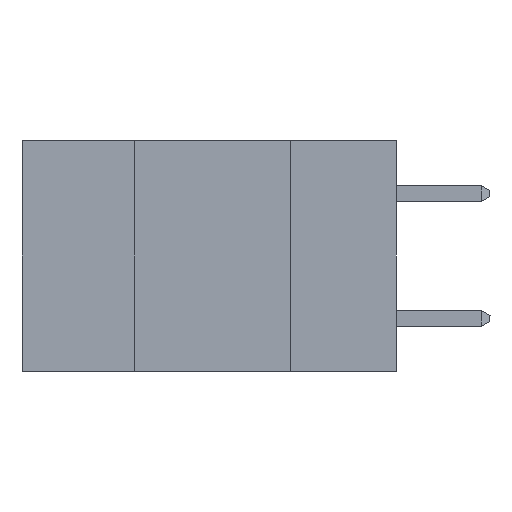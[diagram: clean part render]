
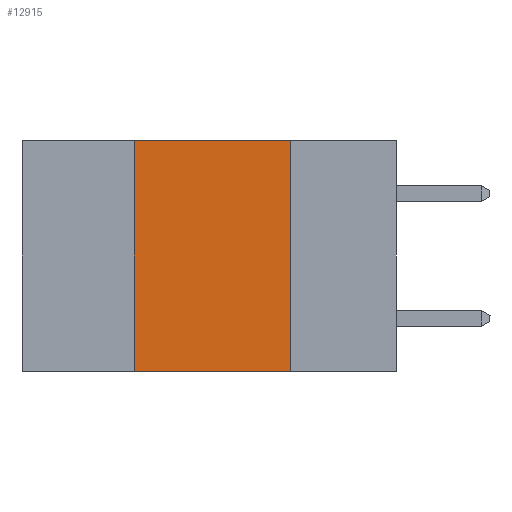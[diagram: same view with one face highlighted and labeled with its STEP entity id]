
A CAD part, left-side view. The second image highlights one B-rep face of the part: STEP entity #12915.
In plain terms, the highlighted planar face has unit normal (-1, 0, 0).
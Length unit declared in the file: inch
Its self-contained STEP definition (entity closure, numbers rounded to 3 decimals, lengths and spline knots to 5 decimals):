
#560 = LINE ( 'NONE', #1571, #10135 ) ;
#811 = LINE ( 'NONE', #8691, #4761 ) ;
#1571 = CARTESIAN_POINT ( 'NONE',  ( 0., 0.17, -0.37 ) ) ;
#2746 = CARTESIAN_POINT ( 'NONE',  ( 0., 0.42, -0.37 ) ) ;
#2854 = CARTESIAN_POINT ( 'NONE',  ( 0., 0.6, 0. ) ) ;
#3634 = CARTESIAN_POINT ( 'NONE',  ( 0., 0.42, -0.37 ) ) ;
#4531 = DIRECTION ( 'NONE',  ( 1., 0., 0. ) ) ;
#4761 = VECTOR ( 'NONE', #20352, 39.37008 ) ;
#5045 = VERTEX_POINT ( 'NONE', #3634 ) ;
#6874 = VECTOR ( 'NONE', #18317, 39.37008 ) ;
#7481 = AXIS2_PLACEMENT_3D ( 'NONE', #2854, #4531, #16347 ) ;
#7601 = ORIENTED_EDGE ( 'NONE', *, *, #12372, .F. ) ;
#8161 = EDGE_CURVE ( 'NONE', #5045, #19670, #811, .T. ) ;
#8289 = CARTESIAN_POINT ( 'NONE',  ( 0., 0.6, 0. ) ) ;
#8691 = CARTESIAN_POINT ( 'NONE',  ( 0., 0.6, -0.37 ) ) ;
#9006 = EDGE_LOOP ( 'NONE', ( #10277, #7601, #13967, #11859 ) ) ;
#10135 = VECTOR ( 'NONE', #13445, 39.37008 ) ;
#10277 = ORIENTED_EDGE ( 'NONE', *, *, #17375, .F. ) ;
#11007 = VERTEX_POINT ( 'NONE', #18142 ) ;
#11859 = ORIENTED_EDGE ( 'NONE', *, *, #8161, .T. ) ;
#12372 = EDGE_CURVE ( 'NONE', #11007, #20914, #20216, .T. ) ;
#12915 = ADVANCED_FACE ( 'NONE', ( #19469 ), #13034, .F. ) ;
#12919 = DIRECTION ( 'NONE',  ( 0., 0., 1. ) ) ;
#13034 = PLANE ( 'NONE',  #7481 ) ;
#13445 = DIRECTION ( 'NONE',  ( 0., 0., -1. ) ) ;
#13967 = ORIENTED_EDGE ( 'NONE', *, *, #15557, .F. ) ;
#14410 = CARTESIAN_POINT ( 'NONE',  ( 0., 0.17, -0.37 ) ) ;
#14467 = VECTOR ( 'NONE', #12919, 39.37008 ) ;
#15557 = EDGE_CURVE ( 'NONE', #5045, #11007, #19863, .T. ) ;
#15920 = CARTESIAN_POINT ( 'NONE',  ( 0., 0.17, 0. ) ) ;
#16347 = DIRECTION ( 'NONE',  ( 0., 0., -1. ) ) ;
#17375 = EDGE_CURVE ( 'NONE', #20914, #19670, #560, .T. ) ;
#18142 = CARTESIAN_POINT ( 'NONE',  ( 0., 0.42, 0. ) ) ;
#18317 = DIRECTION ( 'NONE',  ( 0., -1., 0. ) ) ;
#19469 = FACE_OUTER_BOUND ( 'NONE', #9006, .T. ) ;
#19670 = VERTEX_POINT ( 'NONE', #14410 ) ;
#19863 = LINE ( 'NONE', #2746, #14467 ) ;
#20216 = LINE ( 'NONE', #8289, #6874 ) ;
#20352 = DIRECTION ( 'NONE',  ( 0., -1., 0. ) ) ;
#20914 = VERTEX_POINT ( 'NONE', #15920 ) ;
